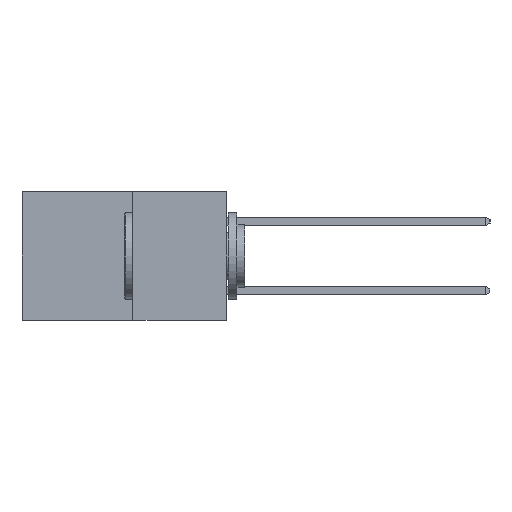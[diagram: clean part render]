
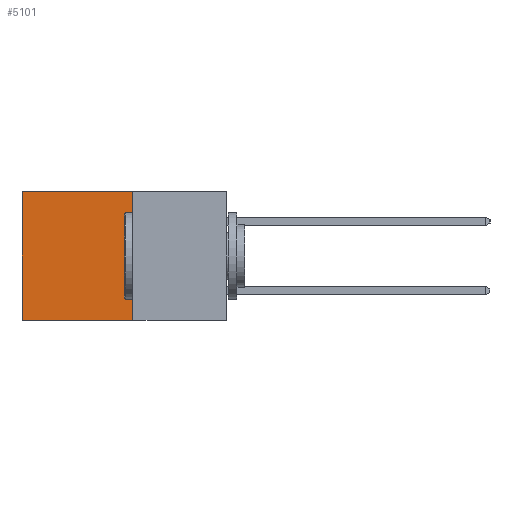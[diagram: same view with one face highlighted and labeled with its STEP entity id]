
A CAD part, left-side view. The second image highlights one B-rep face of the part: STEP entity #5101.
In plain terms, the highlighted planar face has unit normal (-1, 0, 0).
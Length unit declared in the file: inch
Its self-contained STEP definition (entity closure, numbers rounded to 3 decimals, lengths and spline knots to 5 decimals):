
#178 = DIRECTION ( 'NONE',  ( 0., 1., 0. ) ) ;
#346 = CARTESIAN_POINT ( 'NONE',  ( 0.277, 0.27, 0. ) ) ;
#598 = VERTEX_POINT ( 'NONE', #9069 ) ;
#811 = FACE_OUTER_BOUND ( 'NONE', #2186, .T. ) ;
#824 = AXIS2_PLACEMENT_3D ( 'NONE', #1104, #5111, #5550 ) ;
#1104 = CARTESIAN_POINT ( 'NONE',  ( 0.277, 0.27, -0.37 ) ) ;
#1129 = VECTOR ( 'NONE', #178, 39.37008 ) ;
#1267 = LINE ( 'NONE', #7654, #8834 ) ;
#1286 = PLANE ( 'NONE',  #824 ) ;
#1397 = LINE ( 'NONE', #346, #1129 ) ;
#1594 = ORIENTED_EDGE ( 'NONE', *, *, #6462, .T. ) ;
#1622 = VECTOR ( 'NONE', #7248, 39.37008 ) ;
#1735 = DIRECTION ( 'NONE',  ( 0., 1., 0. ) ) ;
#2135 = EDGE_CURVE ( 'NONE', #598, #6874, #1267, .T. ) ;
#2186 = EDGE_LOOP ( 'NONE', ( #5629, #7498, #9077, #1594 ) ) ;
#2350 = VERTEX_POINT ( 'NONE', #8682 ) ;
#2370 = VECTOR ( 'NONE', #2619, 39.37008 ) ;
#2555 = CARTESIAN_POINT ( 'NONE',  ( 0.277, 0.27, -0.37 ) ) ;
#2619 = DIRECTION ( 'NONE',  ( 0., 0., -1. ) ) ;
#3602 = EDGE_CURVE ( 'NONE', #7266, #598, #5880, .T. ) ;
#4051 = EDGE_CURVE ( 'NONE', #2350, #6874, #8238, .T. ) ;
#4876 = CARTESIAN_POINT ( 'NONE',  ( 0.277, 0.59, -0.37 ) ) ;
#5101 = ADVANCED_FACE ( 'NONE', ( #811 ), #1286, .F. ) ;
#5111 = DIRECTION ( 'NONE',  ( 1., 0., 0. ) ) ;
#5375 = CARTESIAN_POINT ( 'NONE',  ( 0.277, 0.27, 0. ) ) ;
#5550 = DIRECTION ( 'NONE',  ( 0., 0., -1. ) ) ;
#5629 = ORIENTED_EDGE ( 'NONE', *, *, #4051, .T. ) ;
#5663 = CARTESIAN_POINT ( 'NONE',  ( 0.277, 0.59, -0.37 ) ) ;
#5880 = LINE ( 'NONE', #2555, #1622 ) ;
#6462 = EDGE_CURVE ( 'NONE', #7266, #2350, #1397, .T. ) ;
#6874 = VERTEX_POINT ( 'NONE', #5663 ) ;
#7248 = DIRECTION ( 'NONE',  ( 0., 0., -1. ) ) ;
#7266 = VERTEX_POINT ( 'NONE', #5375 ) ;
#7498 = ORIENTED_EDGE ( 'NONE', *, *, #2135, .F. ) ;
#7654 = CARTESIAN_POINT ( 'NONE',  ( 0.277, 0.27, -0.37 ) ) ;
#8238 = LINE ( 'NONE', #4876, #2370 ) ;
#8682 = CARTESIAN_POINT ( 'NONE',  ( 0.277, 0.59, 0. ) ) ;
#8834 = VECTOR ( 'NONE', #1735, 39.37008 ) ;
#9069 = CARTESIAN_POINT ( 'NONE',  ( 0.277, 0.27, -0.37 ) ) ;
#9077 = ORIENTED_EDGE ( 'NONE', *, *, #3602, .F. ) ;
